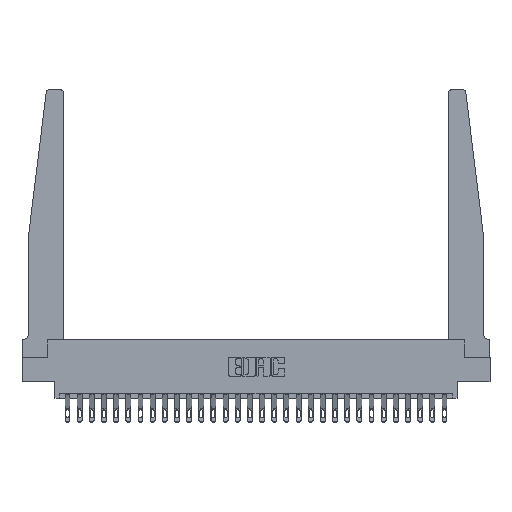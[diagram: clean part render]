
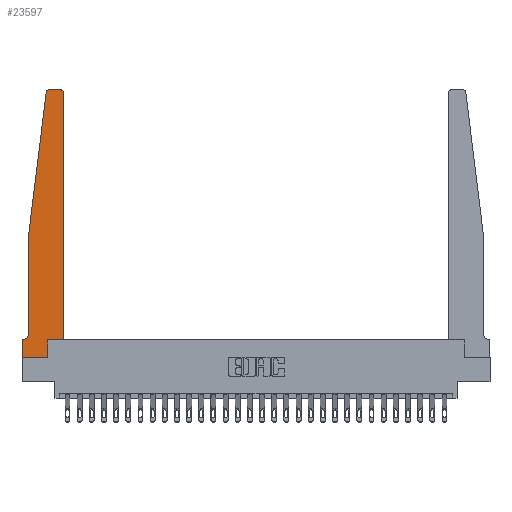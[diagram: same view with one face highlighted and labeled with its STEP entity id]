
A CAD part, top view. The second image highlights one B-rep face of the part: STEP entity #23597.
In plain terms, the highlighted planar face has unit normal (0, 0, 1).
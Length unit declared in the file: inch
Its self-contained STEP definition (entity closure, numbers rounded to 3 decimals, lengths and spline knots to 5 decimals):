
#10 = EDGE_CURVE ( 'NONE', #27839, #13723, #2474, .T. ) ;
#55 = DIRECTION ( 'NONE',  ( -1., 0., 0. ) ) ;
#119 = EDGE_CURVE ( 'NONE', #3292, #15027, #17274, .T. ) ;
#490 = ORIENTED_EDGE ( 'NONE', *, *, #119, .T. ) ;
#494 = CARTESIAN_POINT ( 'NONE',  ( 0.27653, 2.75, 0.37 ) ) ;
#1156 = DIRECTION ( 'NONE',  ( 0., 0., 1. ) ) ;
#1600 = VECTOR ( 'NONE', #14347, 39.37008 ) ;
#1611 = EDGE_CURVE ( 'NONE', #3493, #20256, #9683, .T. ) ;
#2322 = CARTESIAN_POINT ( 'NONE',  ( 0.015, 0.2375, 0.37 ) ) ;
#2474 = LINE ( 'NONE', #21816, #1600 ) ;
#2478 = LINE ( 'NONE', #19973, #7054 ) ;
#2656 = DIRECTION ( 'NONE',  ( 1., 0., 0. ) ) ;
#2985 = DIRECTION ( 'NONE',  ( 1., 0., 0. ) ) ;
#3015 = ORIENTED_EDGE ( 'NONE', *, *, #7476, .T. ) ;
#3073 = AXIS2_PLACEMENT_3D ( 'NONE', #24891, #1156, #25183 ) ;
#3292 = VERTEX_POINT ( 'NONE', #13332 ) ;
#3493 = VERTEX_POINT ( 'NONE', #18816 ) ;
#4427 = EDGE_CURVE ( 'NONE', #25751, #12789, #12692, .T. ) ;
#5441 = ORIENTED_EDGE ( 'NONE', *, *, #10, .T. ) ;
#5452 = ORIENTED_EDGE ( 'NONE', *, *, #21393, .T. ) ;
#5750 = DIRECTION ( 'NONE',  ( -1., 0., 0. ) ) ;
#6131 = CARTESIAN_POINT ( 'NONE',  ( 0.065, 1.25, 0.37 ) ) ;
#6726 = DIRECTION ( 'NONE',  ( 0., 0., 1. ) ) ;
#6843 = AXIS2_PLACEMENT_3D ( 'NONE', #26367, #6726, #2656 ) ;
#6913 = VERTEX_POINT ( 'NONE', #494 ) ;
#7054 = VECTOR ( 'NONE', #9094, 39.37008 ) ;
#7476 = EDGE_CURVE ( 'NONE', #6913, #24481, #24726, .T. ) ;
#7537 = CARTESIAN_POINT ( 'NONE',  ( 0., 0., 0.37 ) ) ;
#9094 = DIRECTION ( 'NONE',  ( -1., 0., 0. ) ) ;
#9106 = EDGE_LOOP ( 'NONE', ( #20818, #3015, #5452, #490, #22689, #18939, #5441, #12109, #11651, #17117, #15175, #24427 ) ) ;
#9683 = LINE ( 'NONE', #18282, #21016 ) ;
#9869 = FACE_OUTER_BOUND ( 'NONE', #9106, .T. ) ;
#10213 = LINE ( 'NONE', #25352, #20148 ) ;
#10639 = DIRECTION ( 'NONE',  ( -0.122, -0.992, 0. ) ) ;
#10968 = CARTESIAN_POINT ( 'NONE',  ( 0.395, 2.75, 0.37 ) ) ;
#11189 = CARTESIAN_POINT ( 'NONE',  ( 0., 0.1875, 0.37 ) ) ;
#11514 = VERTEX_POINT ( 'NONE', #18882 ) ;
#11651 = ORIENTED_EDGE ( 'NONE', *, *, #1611, .T. ) ;
#12109 = ORIENTED_EDGE ( 'NONE', *, *, #14585, .T. ) ;
#12586 = CIRCLE ( 'NONE', #17991, 0.05 ) ;
#12600 = DIRECTION ( 'NONE',  ( 1., 0., 0. ) ) ;
#12679 = CARTESIAN_POINT ( 'NONE',  ( 0.425, 0.18, 0.37 ) ) ;
#12692 = CIRCLE ( 'NONE', #6843, 0.03 ) ;
#12750 = DIRECTION ( 'NONE',  ( 0., 0., -1. ) ) ;
#12789 = VERTEX_POINT ( 'NONE', #10968 ) ;
#13332 = CARTESIAN_POINT ( 'NONE',  ( 0.065, 1.25, 0.37 ) ) ;
#13423 = CARTESIAN_POINT ( 'NONE',  ( 0., 0., 0.37 ) ) ;
#13723 = VERTEX_POINT ( 'NONE', #13423 ) ;
#13843 = DIRECTION ( 'NONE',  ( 0., 1., 0. ) ) ;
#13904 = VERTEX_POINT ( 'NONE', #12679 ) ;
#14019 = CARTESIAN_POINT ( 'NONE',  ( 0.425, 2.72, 0.37 ) ) ;
#14238 = VECTOR ( 'NONE', #24913, 39.37008 ) ;
#14347 = DIRECTION ( 'NONE',  ( 0., -1., 0. ) ) ;
#14585 = EDGE_CURVE ( 'NONE', #13723, #3493, #26888, .T. ) ;
#14899 = CARTESIAN_POINT ( 'NONE',  ( 0.24675, 2.72367, 0.37 ) ) ;
#15027 = VERTEX_POINT ( 'NONE', #22738 ) ;
#15159 = CARTESIAN_POINT ( 'NONE',  ( 0.065, 1.25, 0.37 ) ) ;
#15175 = ORIENTED_EDGE ( 'NONE', *, *, #16153, .T. ) ;
#15932 = PLANE ( 'NONE',  #24358 ) ;
#16153 = EDGE_CURVE ( 'NONE', #13904, #25751, #26445, .T. ) ;
#16961 = VECTOR ( 'NONE', #10639, 39.37008 ) ;
#17117 = ORIENTED_EDGE ( 'NONE', *, *, #21712, .T. ) ;
#17274 = LINE ( 'NONE', #15159, #26865 ) ;
#17937 = CARTESIAN_POINT ( 'NONE',  ( 0.425, 0.18, 0.37 ) ) ;
#17991 = AXIS2_PLACEMENT_3D ( 'NONE', #2322, #12750, #55 ) ;
#18060 = CARTESIAN_POINT ( 'NONE',  ( 0., 0.1875, 0.37 ) ) ;
#18282 = CARTESIAN_POINT ( 'NONE',  ( 0.2605, 0.18, 0.37 ) ) ;
#18698 = VECTOR ( 'NONE', #13843, 39.37008 ) ;
#18816 = CARTESIAN_POINT ( 'NONE',  ( 0.2605, 0., 0.37 ) ) ;
#18882 = CARTESIAN_POINT ( 'NONE',  ( 0.015, 0.1875, 0.37 ) ) ;
#18939 = ORIENTED_EDGE ( 'NONE', *, *, #21537, .T. ) ;
#19053 = CARTESIAN_POINT ( 'NONE',  ( 0.2605, 0.18, 0.37 ) ) ;
#19973 = CARTESIAN_POINT ( 'NONE',  ( 0.065, 0.1875, 0.37 ) ) ;
#20148 = VECTOR ( 'NONE', #12600, 39.37008 ) ;
#20256 = VERTEX_POINT ( 'NONE', #19053 ) ;
#20818 = ORIENTED_EDGE ( 'NONE', *, *, #25603, .T. ) ;
#21016 = VECTOR ( 'NONE', #26918, 39.37008 ) ;
#21157 = CARTESIAN_POINT ( 'NONE',  ( 0.25, 2.75, 0.37 ) ) ;
#21393 = EDGE_CURVE ( 'NONE', #24481, #3292, #21405, .T. ) ;
#21405 = LINE ( 'NONE', #6131, #16961 ) ;
#21537 = EDGE_CURVE ( 'NONE', #11514, #27839, #2478, .T. ) ;
#21712 = EDGE_CURVE ( 'NONE', #20256, #13904, #10213, .T. ) ;
#21816 = CARTESIAN_POINT ( 'NONE',  ( 0., 0., 0.37 ) ) ;
#22689 = ORIENTED_EDGE ( 'NONE', *, *, #24878, .T. ) ;
#22738 = CARTESIAN_POINT ( 'NONE',  ( 0.065, 0.2375, 0.37 ) ) ;
#23597 = ADVANCED_FACE ( 'NONE', ( #9869 ), #15932, .T. ) ;
#23806 = DIRECTION ( 'NONE',  ( 0., -1., 0. ) ) ;
#24358 = AXIS2_PLACEMENT_3D ( 'NONE', #18060, #26559, #2985 ) ;
#24427 = ORIENTED_EDGE ( 'NONE', *, *, #4427, .T. ) ;
#24481 = VERTEX_POINT ( 'NONE', #14899 ) ;
#24726 = CIRCLE ( 'NONE', #3073, 0.03 ) ;
#24878 = EDGE_CURVE ( 'NONE', #15027, #11514, #12586, .T. ) ;
#24891 = CARTESIAN_POINT ( 'NONE',  ( 0.27653, 2.72, 0.37 ) ) ;
#24913 = DIRECTION ( 'NONE',  ( 1., 0., 0. ) ) ;
#25183 = DIRECTION ( 'NONE',  ( 1., 0., 0. ) ) ;
#25273 = VECTOR ( 'NONE', #5750, 39.37008 ) ;
#25352 = CARTESIAN_POINT ( 'NONE',  ( 0.425, 0.18, 0.37 ) ) ;
#25603 = EDGE_CURVE ( 'NONE', #12789, #6913, #27226, .T. ) ;
#25751 = VERTEX_POINT ( 'NONE', #14019 ) ;
#26367 = CARTESIAN_POINT ( 'NONE',  ( 0.395, 2.72, 0.37 ) ) ;
#26445 = LINE ( 'NONE', #17937, #18698 ) ;
#26559 = DIRECTION ( 'NONE',  ( 0., 0., 1. ) ) ;
#26865 = VECTOR ( 'NONE', #23806, 39.37008 ) ;
#26888 = LINE ( 'NONE', #7537, #14238 ) ;
#26918 = DIRECTION ( 'NONE',  ( 0., 1., 0. ) ) ;
#27226 = LINE ( 'NONE', #21157, #25273 ) ;
#27839 = VERTEX_POINT ( 'NONE', #11189 ) ;
